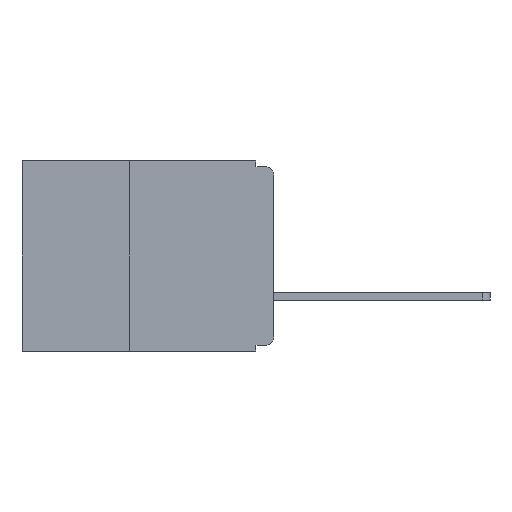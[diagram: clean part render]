
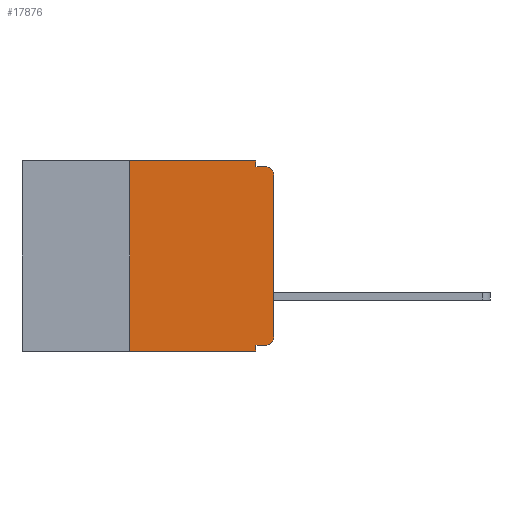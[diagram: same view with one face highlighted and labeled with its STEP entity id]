
A CAD part, left-side view. The second image highlights one B-rep face of the part: STEP entity #17876.
In plain terms, the highlighted planar face has unit normal (-1, 0, 0).
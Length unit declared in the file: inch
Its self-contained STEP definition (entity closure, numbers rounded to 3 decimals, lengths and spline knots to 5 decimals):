
#61 = DIRECTION ( 'NONE',  ( 0., -1., 0. ) ) ;
#168 = VECTOR ( 'NONE', #11708, 39.37008 ) ;
#217 = LINE ( 'NONE', #11889, #168 ) ;
#536 = LINE ( 'NONE', #12577, #624 ) ;
#624 = VECTOR ( 'NONE', #12489, 39.37008 ) ;
#808 = EDGE_CURVE ( 'NONE', #5160, #6404, #1752, .T. ) ;
#1752 = CIRCLE ( 'NONE', #7426, 0.015 ) ;
#1806 = CARTESIAN_POINT ( 'NONE',  ( 0., 0.015, -0.32 ) ) ;
#2219 = EDGE_CURVE ( 'NONE', #8983, #6306, #5437, .T. ) ;
#2420 = ORIENTED_EDGE ( 'NONE', *, *, #12439, .T. ) ;
#2597 = VERTEX_POINT ( 'NONE', #10813 ) ;
#3394 = DIRECTION ( 'NONE',  ( 0., 0., -1. ) ) ;
#3415 = CARTESIAN_POINT ( 'NONE',  ( 0., 0.031, -0.01 ) ) ;
#3540 = CARTESIAN_POINT ( 'NONE',  ( 0., 0.437, -0.33 ) ) ;
#3585 = ORIENTED_EDGE ( 'NONE', *, *, #13727, .F. ) ;
#4315 = ORIENTED_EDGE ( 'NONE', *, *, #16393, .F. ) ;
#4418 = DIRECTION ( 'NONE',  ( 0., -1., 0. ) ) ;
#4540 = VERTEX_POINT ( 'NONE', #3415 ) ;
#4640 = CIRCLE ( 'NONE', #7262, 0.015 ) ;
#4787 = ORIENTED_EDGE ( 'NONE', *, *, #808, .T. ) ;
#4845 = EDGE_CURVE ( 'NONE', #6306, #4540, #16381, .T. ) ;
#4910 = ORIENTED_EDGE ( 'NONE', *, *, #5807, .F. ) ;
#5037 = VECTOR ( 'NONE', #10992, 39.37008 ) ;
#5160 = VERTEX_POINT ( 'NONE', #1806 ) ;
#5216 = LINE ( 'NONE', #14125, #5037 ) ;
#5331 = VECTOR ( 'NONE', #4418, 39.37008 ) ;
#5437 = LINE ( 'NONE', #9429, #5331 ) ;
#5807 = EDGE_CURVE ( 'NONE', #8561, #8983, #10756, .T. ) ;
#6204 = ORIENTED_EDGE ( 'NONE', *, *, #4845, .F. ) ;
#6306 = VERTEX_POINT ( 'NONE', #17141 ) ;
#6404 = VERTEX_POINT ( 'NONE', #12620 ) ;
#6510 = DIRECTION ( 'NONE',  ( 0., 0., -1. ) ) ;
#6571 = CARTESIAN_POINT ( 'NONE',  ( 0., 0.25, 0. ) ) ;
#6578 = DIRECTION ( 'NONE',  ( 1., 0., 0. ) ) ;
#6774 = AXIS2_PLACEMENT_3D ( 'NONE', #7232, #6578, #6510 ) ;
#6794 = ORIENTED_EDGE ( 'NONE', *, *, #10823, .F. ) ;
#6896 = PLANE ( 'NONE',  #6774 ) ;
#6976 = VECTOR ( 'NONE', #61, 39.37008 ) ;
#7015 = LINE ( 'NONE', #3540, #6976 ) ;
#7070 = ORIENTED_EDGE ( 'NONE', *, *, #2219, .F. ) ;
#7232 = CARTESIAN_POINT ( 'NONE',  ( 0., 0.437, 0. ) ) ;
#7262 = AXIS2_PLACEMENT_3D ( 'NONE', #15560, #15522, #15467 ) ;
#7426 = AXIS2_PLACEMENT_3D ( 'NONE', #16066, #16118, #3394 ) ;
#7548 = DIRECTION ( 'NONE',  ( 0., 0., 1. ) ) ;
#7558 = FACE_OUTER_BOUND ( 'NONE', #14209, .T. ) ;
#7628 = VERTEX_POINT ( 'NONE', #12608 ) ;
#7653 = CARTESIAN_POINT ( 'NONE',  ( 0., 0., 0. ) ) ;
#8341 = VECTOR ( 'NONE', #7548, 39.37008 ) ;
#8561 = VERTEX_POINT ( 'NONE', #17276 ) ;
#8659 = CARTESIAN_POINT ( 'NONE',  ( 0., 0.015, -0.01 ) ) ;
#8983 = VERTEX_POINT ( 'NONE', #6571 ) ;
#9429 = CARTESIAN_POINT ( 'NONE',  ( 0., 0.437, 0. ) ) ;
#9824 = VERTEX_POINT ( 'NONE', #8659 ) ;
#9870 = EDGE_CURVE ( 'NONE', #6404, #7628, #10195, .T. ) ;
#10195 = LINE ( 'NONE', #7653, #8341 ) ;
#10723 = VECTOR ( 'NONE', #14342, 39.37008 ) ;
#10756 = LINE ( 'NONE', #14549, #10723 ) ;
#10764 = ORIENTED_EDGE ( 'NONE', *, *, #9870, .T. ) ;
#10813 = CARTESIAN_POINT ( 'NONE',  ( 0., 0.031, -0.32 ) ) ;
#10823 = EDGE_CURVE ( 'NONE', #5160, #2597, #217, .T. ) ;
#10992 = DIRECTION ( 'NONE',  ( 0., -1., 0. ) ) ;
#11031 = CARTESIAN_POINT ( 'NONE',  ( 0., 0.031, -0.33 ) ) ;
#11708 = DIRECTION ( 'NONE',  ( 0., 1., 0. ) ) ;
#11889 = CARTESIAN_POINT ( 'NONE',  ( 0., 0., -0.32 ) ) ;
#12439 = EDGE_CURVE ( 'NONE', #8561, #13789, #7015, .T. ) ;
#12489 = DIRECTION ( 'NONE',  ( 0., 0., -1. ) ) ;
#12577 = CARTESIAN_POINT ( 'NONE',  ( 0., 0.031, -0.33 ) ) ;
#12608 = CARTESIAN_POINT ( 'NONE',  ( 0., 0., -0.025 ) ) ;
#12620 = CARTESIAN_POINT ( 'NONE',  ( 0., 0., -0.305 ) ) ;
#13727 = EDGE_CURVE ( 'NONE', #2597, #13789, #536, .T. ) ;
#13789 = VERTEX_POINT ( 'NONE', #11031 ) ;
#14125 = CARTESIAN_POINT ( 'NONE',  ( 0., 0., -0.01 ) ) ;
#14209 = EDGE_LOOP ( 'NONE', ( #10764, #14537, #4315, #6204, #7070, #4910, #2420, #3585, #6794, #4787 ) ) ;
#14342 = DIRECTION ( 'NONE',  ( 0., 0., 1. ) ) ;
#14537 = ORIENTED_EDGE ( 'NONE', *, *, #16459, .T. ) ;
#14549 = CARTESIAN_POINT ( 'NONE',  ( 0., 0.25, -0.33 ) ) ;
#15158 = DIRECTION ( 'NONE',  ( 0., 0., -1. ) ) ;
#15339 = CARTESIAN_POINT ( 'NONE',  ( 0., 0.031, 0. ) ) ;
#15467 = DIRECTION ( 'NONE',  ( 0., 0., -1. ) ) ;
#15522 = DIRECTION ( 'NONE',  ( -1., 0., 0. ) ) ;
#15560 = CARTESIAN_POINT ( 'NONE',  ( 0., 0.015, -0.025 ) ) ;
#16066 = CARTESIAN_POINT ( 'NONE',  ( 0., 0.015, -0.305 ) ) ;
#16118 = DIRECTION ( 'NONE',  ( -1., 0., 0. ) ) ;
#16327 = VECTOR ( 'NONE', #15158, 39.37008 ) ;
#16381 = LINE ( 'NONE', #15339, #16327 ) ;
#16393 = EDGE_CURVE ( 'NONE', #4540, #9824, #5216, .T. ) ;
#16459 = EDGE_CURVE ( 'NONE', #7628, #9824, #4640, .T. ) ;
#17141 = CARTESIAN_POINT ( 'NONE',  ( 0., 0.031, 0. ) ) ;
#17276 = CARTESIAN_POINT ( 'NONE',  ( 0., 0.25, -0.33 ) ) ;
#17876 = ADVANCED_FACE ( 'NONE', ( #7558 ), #6896, .F. ) ;
